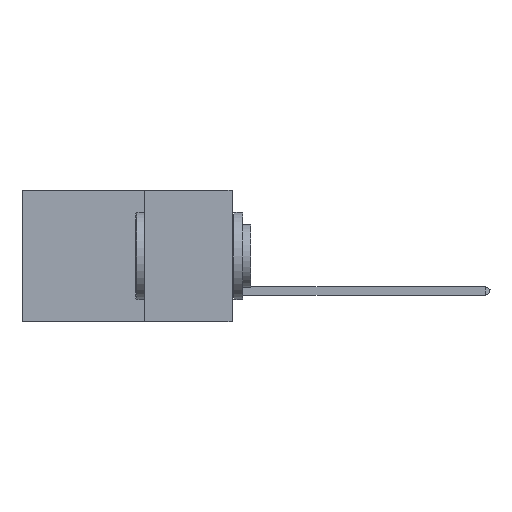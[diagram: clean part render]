
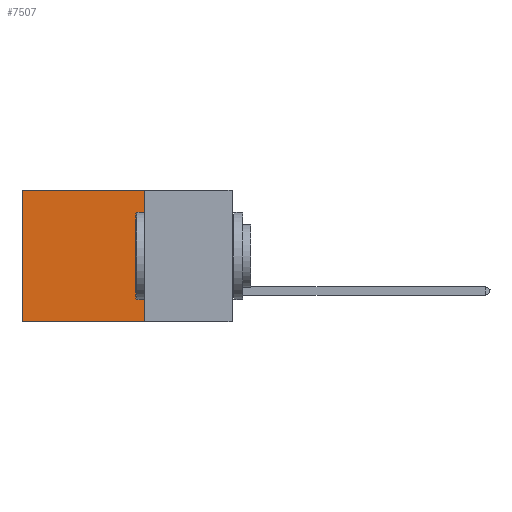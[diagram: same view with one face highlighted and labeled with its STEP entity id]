
A CAD part, left-side view. The second image highlights one B-rep face of the part: STEP entity #7507.
In plain terms, the highlighted planar face has unit normal (-1, 0, 0).
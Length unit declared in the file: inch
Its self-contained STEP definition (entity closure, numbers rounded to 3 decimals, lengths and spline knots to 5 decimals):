
#417 = CARTESIAN_POINT ( 'NONE',  ( 0.2875, 0.6, 0. ) ) ;
#1266 = VERTEX_POINT ( 'NONE', #10971 ) ;
#1908 = LINE ( 'NONE', #21285, #15179 ) ;
#2181 = EDGE_CURVE ( 'NONE', #1266, #15723, #8748, .T. ) ;
#2781 = DIRECTION ( 'NONE',  ( 1., 0., 0. ) ) ;
#3355 = DIRECTION ( 'NONE',  ( 0., 0., -1. ) ) ;
#5720 = VECTOR ( 'NONE', #16760, 39.37008 ) ;
#7002 = LINE ( 'NONE', #8323, #15324 ) ;
#7014 = ORIENTED_EDGE ( 'NONE', *, *, #19126, .T. ) ;
#7507 = ADVANCED_FACE ( 'NONE', ( #15619 ), #7826, .F. ) ;
#7680 = VERTEX_POINT ( 'NONE', #13332 ) ;
#7826 = PLANE ( 'NONE',  #13134 ) ;
#8323 = CARTESIAN_POINT ( 'NONE',  ( 0.2875, 0.25, -0.375 ) ) ;
#8748 = LINE ( 'NONE', #17851, #21228 ) ;
#9313 = VERTEX_POINT ( 'NONE', #18819 ) ;
#10971 = CARTESIAN_POINT ( 'NONE',  ( 0.2875, 0.25, 0. ) ) ;
#12723 = LINE ( 'NONE', #18283, #5720 ) ;
#13134 = AXIS2_PLACEMENT_3D ( 'NONE', #17563, #2781, #14279 ) ;
#13332 = CARTESIAN_POINT ( 'NONE',  ( 0.2875, 0.6, -0.375 ) ) ;
#13793 = EDGE_CURVE ( 'NONE', #1266, #9313, #7002, .T. ) ;
#14279 = DIRECTION ( 'NONE',  ( 0., 0., -1. ) ) ;
#14460 = ORIENTED_EDGE ( 'NONE', *, *, #17194, .F. ) ;
#15179 = VECTOR ( 'NONE', #19545, 39.37008 ) ;
#15324 = VECTOR ( 'NONE', #3355, 39.37008 ) ;
#15619 = FACE_OUTER_BOUND ( 'NONE', #18058, .T. ) ;
#15723 = VERTEX_POINT ( 'NONE', #417 ) ;
#16760 = DIRECTION ( 'NONE',  ( 0., 0., -1. ) ) ;
#17194 = EDGE_CURVE ( 'NONE', #9313, #7680, #1908, .T. ) ;
#17563 = CARTESIAN_POINT ( 'NONE',  ( 0.2875, 0.25, -0.375 ) ) ;
#17631 = ORIENTED_EDGE ( 'NONE', *, *, #13793, .F. ) ;
#17782 = DIRECTION ( 'NONE',  ( 0., 1., 0. ) ) ;
#17851 = CARTESIAN_POINT ( 'NONE',  ( 0.2875, 0.25, 0. ) ) ;
#18004 = ORIENTED_EDGE ( 'NONE', *, *, #2181, .T. ) ;
#18058 = EDGE_LOOP ( 'NONE', ( #7014, #14460, #17631, #18004 ) ) ;
#18283 = CARTESIAN_POINT ( 'NONE',  ( 0.2875, 0.6, -0.375 ) ) ;
#18819 = CARTESIAN_POINT ( 'NONE',  ( 0.2875, 0.25, -0.375 ) ) ;
#19126 = EDGE_CURVE ( 'NONE', #15723, #7680, #12723, .T. ) ;
#19545 = DIRECTION ( 'NONE',  ( 0., 1., 0. ) ) ;
#21228 = VECTOR ( 'NONE', #17782, 39.37008 ) ;
#21285 = CARTESIAN_POINT ( 'NONE',  ( 0.2875, 0.25, -0.375 ) ) ;
